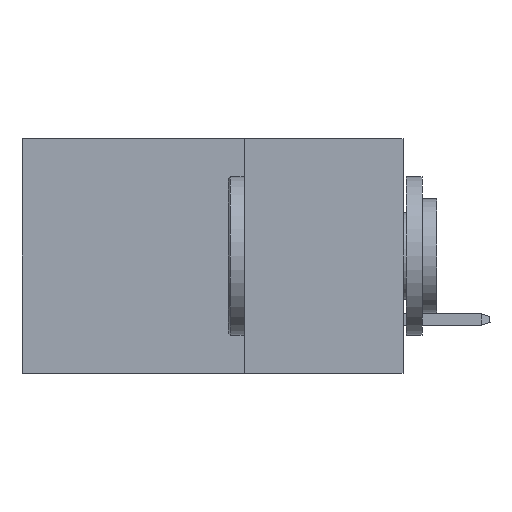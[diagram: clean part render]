
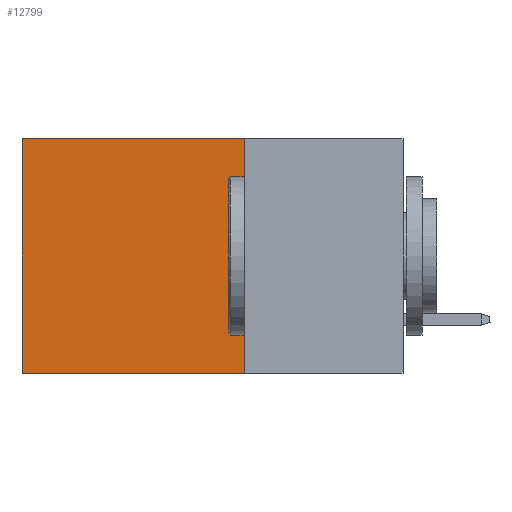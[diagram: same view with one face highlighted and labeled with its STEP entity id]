
A CAD part, left-side view. The second image highlights one B-rep face of the part: STEP entity #12799.
In plain terms, the highlighted planar face has unit normal (-1, 0, 0).
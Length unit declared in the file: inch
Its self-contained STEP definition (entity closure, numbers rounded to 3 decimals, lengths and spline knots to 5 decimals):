
#1717 = EDGE_CURVE ( 'NONE', #8275, #18547, #28754, .T. ) ;
#2315 = DIRECTION ( 'NONE',  ( 1., 0., 0. ) ) ;
#2362 = VERTEX_POINT ( 'NONE', #16255 ) ;
#3801 = CARTESIAN_POINT ( 'NONE',  ( 0.2875, 0.25, -0.37 ) ) ;
#3826 = CARTESIAN_POINT ( 'NONE',  ( 0.2875, 0.6, 0. ) ) ;
#4380 = ORIENTED_EDGE ( 'NONE', *, *, #1717, .F. ) ;
#5377 = CARTESIAN_POINT ( 'NONE',  ( 0.2875, 0.25, 0. ) ) ;
#5580 = ORIENTED_EDGE ( 'NONE', *, *, #19269, .T. ) ;
#8275 = VERTEX_POINT ( 'NONE', #36894 ) ;
#12799 = ADVANCED_FACE ( 'NONE', ( #23984 ), #32868, .F. ) ;
#13427 = LINE ( 'NONE', #28644, #18114 ) ;
#13671 = EDGE_CURVE ( 'NONE', #18547, #2362, #25755, .T. ) ;
#13863 = VECTOR ( 'NONE', #35437, 39.37008 ) ;
#14597 = DIRECTION ( 'NONE',  ( 0., 0., -1. ) ) ;
#14616 = LINE ( 'NONE', #26829, #26296 ) ;
#15462 = ORIENTED_EDGE ( 'NONE', *, *, #13671, .F. ) ;
#16255 = CARTESIAN_POINT ( 'NONE',  ( 0.2875, 0.6, -0.37 ) ) ;
#16438 = DIRECTION ( 'NONE',  ( 0., 0., -1. ) ) ;
#17637 = VECTOR ( 'NONE', #38265, 39.37008 ) ;
#18114 = VECTOR ( 'NONE', #16438, 39.37008 ) ;
#18547 = VERTEX_POINT ( 'NONE', #3801 ) ;
#19269 = EDGE_CURVE ( 'NONE', #8275, #33357, #14616, .T. ) ;
#21347 = EDGE_CURVE ( 'NONE', #33357, #2362, #13427, .T. ) ;
#23873 = ORIENTED_EDGE ( 'NONE', *, *, #21347, .T. ) ;
#23984 = FACE_OUTER_BOUND ( 'NONE', #37049, .T. ) ;
#25755 = LINE ( 'NONE', #25958, #17637 ) ;
#25958 = CARTESIAN_POINT ( 'NONE',  ( 0.2875, 0.25, -0.37 ) ) ;
#26296 = VECTOR ( 'NONE', #39356, 39.37008 ) ;
#26829 = CARTESIAN_POINT ( 'NONE',  ( 0.2875, 0.25, 0. ) ) ;
#28644 = CARTESIAN_POINT ( 'NONE',  ( 0.2875, 0.6, 0. ) ) ;
#28754 = LINE ( 'NONE', #28948, #13863 ) ;
#28948 = CARTESIAN_POINT ( 'NONE',  ( 0.2875, 0.25, 0. ) ) ;
#32868 = PLANE ( 'NONE',  #37472 ) ;
#33357 = VERTEX_POINT ( 'NONE', #3826 ) ;
#35437 = DIRECTION ( 'NONE',  ( 0., 0., -1. ) ) ;
#36894 = CARTESIAN_POINT ( 'NONE',  ( 0.2875, 0.25, 0. ) ) ;
#37049 = EDGE_LOOP ( 'NONE', ( #23873, #15462, #4380, #5580 ) ) ;
#37472 = AXIS2_PLACEMENT_3D ( 'NONE', #5377, #2315, #14597 ) ;
#38265 = DIRECTION ( 'NONE',  ( 0., 1., 0. ) ) ;
#39356 = DIRECTION ( 'NONE',  ( 0., 1., 0. ) ) ;
